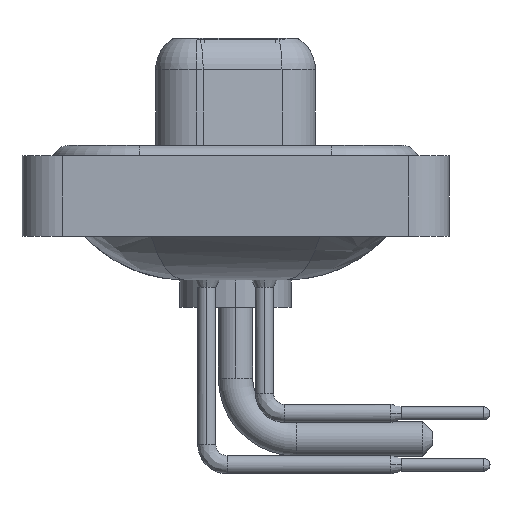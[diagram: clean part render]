
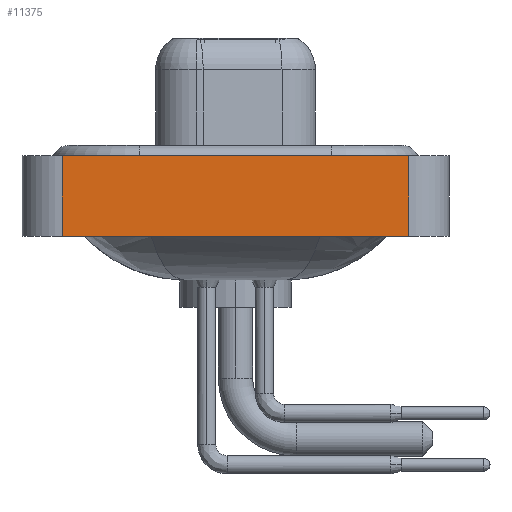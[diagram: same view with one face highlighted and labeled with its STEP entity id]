
A CAD part, left-side view. The second image highlights one B-rep face of the part: STEP entity #11375.
In plain terms, the highlighted planar face has unit normal (-1, 0, 0).
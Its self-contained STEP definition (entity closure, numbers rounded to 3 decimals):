
#130 = CARTESIAN_POINT ( 'NONE',  ( -7.35, -8.55, 0.4 ) ) ;
#182 = VERTEX_POINT ( 'NONE', #1625 ) ;
#549 = VERTEX_POINT ( 'NONE', #25186 ) ;
#764 = VECTOR ( 'NONE', #16225, 1000. ) ;
#1014 = DIRECTION ( 'NONE',  ( 0., 0., 1. ) ) ;
#1625 = CARTESIAN_POINT ( 'NONE',  ( -7.35, -8.55, -3.6 ) ) ;
#1688 = CARTESIAN_POINT ( 'NONE',  ( -7.35, -8.55, -3.6 ) ) ;
#6368 = LINE ( 'NONE', #8101, #764 ) ;
#6922 = CARTESIAN_POINT ( 'NONE',  ( -7.35, 8.55, -3.6 ) ) ;
#8101 = CARTESIAN_POINT ( 'NONE',  ( -7.35, -8.55, -3.6 ) ) ;
#8321 = EDGE_CURVE ( 'NONE', #182, #549, #21564, .T. ) ;
#8645 = CARTESIAN_POINT ( 'NONE',  ( -7.35, 8.55, 0.4 ) ) ;
#9569 = PLANE ( 'NONE',  #16675 ) ;
#9585 = ORIENTED_EDGE ( 'NONE', *, *, #8321, .T. ) ;
#11158 = CARTESIAN_POINT ( 'NONE',  ( -7.35, -8.55, -3.6 ) ) ;
#11375 = ADVANCED_FACE ( 'NONE', ( #17447 ), #9569, .T. ) ;
#11952 = CARTESIAN_POINT ( 'NONE',  ( -7.35, 8.55, -3.6 ) ) ;
#12293 = DIRECTION ( 'NONE',  ( 0., -1., 0. ) ) ;
#12793 = ORIENTED_EDGE ( 'NONE', *, *, #23074, .F. ) ;
#13067 = VECTOR ( 'NONE', #12293, 1000. ) ;
#14074 = DIRECTION ( 'NONE',  ( 0., 0., 1. ) ) ;
#15660 = VECTOR ( 'NONE', #1014, 1000. ) ;
#15954 = LINE ( 'NONE', #11952, #19617 ) ;
#16225 = DIRECTION ( 'NONE',  ( 0., -1., 0. ) ) ;
#16675 = AXIS2_PLACEMENT_3D ( 'NONE', #1688, #19709, #25703 ) ;
#17447 = FACE_OUTER_BOUND ( 'NONE', #24017, .T. ) ;
#19418 = EDGE_CURVE ( 'NONE', #19835, #549, #22567, .T. ) ;
#19617 = VECTOR ( 'NONE', #14074, 1000. ) ;
#19709 = DIRECTION ( 'NONE',  ( -1., 0., 0. ) ) ;
#19835 = VERTEX_POINT ( 'NONE', #8645 ) ;
#20047 = VERTEX_POINT ( 'NONE', #6922 ) ;
#21564 = LINE ( 'NONE', #11158, #15660 ) ;
#21609 = ORIENTED_EDGE ( 'NONE', *, *, #19418, .F. ) ;
#21668 = EDGE_CURVE ( 'NONE', #20047, #182, #6368, .T. ) ;
#22567 = LINE ( 'NONE', #130, #13067 ) ;
#23074 = EDGE_CURVE ( 'NONE', #20047, #19835, #15954, .T. ) ;
#24017 = EDGE_LOOP ( 'NONE', ( #9585, #21609, #12793, #25955 ) ) ;
#25186 = CARTESIAN_POINT ( 'NONE',  ( -7.35, -8.55, 0.4 ) ) ;
#25703 = DIRECTION ( 'NONE',  ( 0., 0., 1. ) ) ;
#25955 = ORIENTED_EDGE ( 'NONE', *, *, #21668, .T. ) ;
